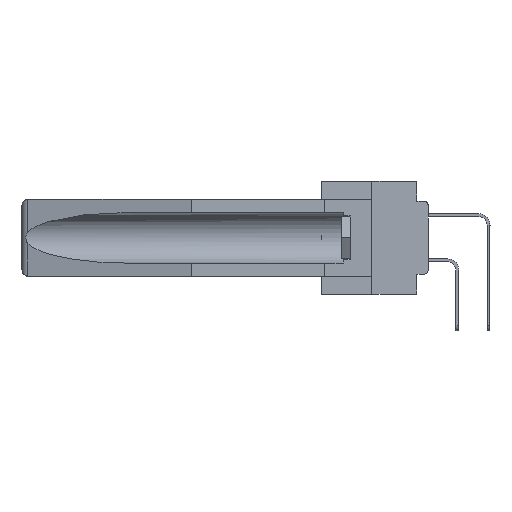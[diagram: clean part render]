
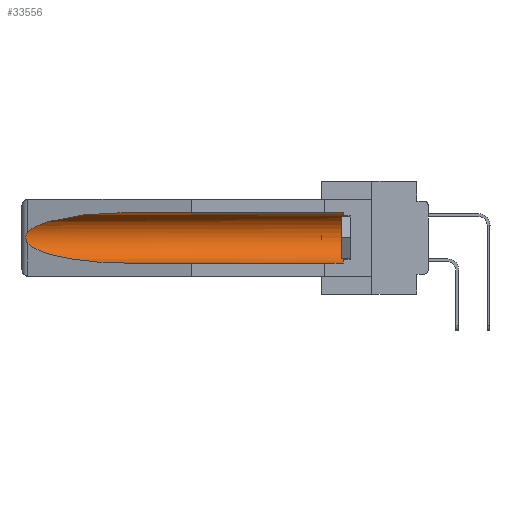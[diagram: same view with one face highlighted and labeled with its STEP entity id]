
A CAD part, left-side view. The second image highlights one B-rep face of the part: STEP entity #33556.
In plain terms, the highlighted cylindrical face has radius 2.857 mm (diameter 5.715 mm), a partial arc.
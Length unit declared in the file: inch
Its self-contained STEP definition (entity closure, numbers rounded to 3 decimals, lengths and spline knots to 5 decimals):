
#697 = DIRECTION ( 'NONE',  ( 0., 0., 1. ) ) ;
#1039 = CARTESIAN_POINT ( 'NONE',  ( 0.155, 1.07973, -0.284 ) ) ;
#2254 = CARTESIAN_POINT ( 'NONE',  ( 0.26537, 1.52718, -0.14972 ) ) ;
#2751 = VERTEX_POINT ( 'NONE', #34469 ) ;
#3448 = CARTESIAN_POINT ( 'NONE',  ( 0.2675, 1.53308, -0.16763 ) ) ;
#3685 = AXIS2_PLACEMENT_3D ( 'NONE', #16820, #39530, #697 ) ;
#3719 = CARTESIAN_POINT ( 'NONE',  ( 0.26654, 1.53092, -0.15636 ) ) ;
#5599 = CYLINDRICAL_SURFACE ( 'NONE', #23525, 0.1125 ) ;
#5653 = CARTESIAN_POINT ( 'NONE',  ( 0.155, -0.30754, -0.284 ) ) ;
#6281 = LINE ( 'NONE', #5653, #39744 ) ;
#6482 = CARTESIAN_POINT ( 'NONE',  ( 0.155, 1.07973, -0.284 ) ) ;
#7135 = VERTEX_POINT ( 'NONE', #21342 ) ;
#7260 = CARTESIAN_POINT ( 'NONE',  ( 0.26537, 1.52718, -0.19328 ) ) ;
#7741 = VERTEX_POINT ( 'NONE', #1039 ) ;
#11062 = EDGE_LOOP ( 'NONE', ( #20081, #21337, #25285, #20345, #12530, #34948 ) ) ;
#11138 =( BOUNDED_CURVE ( )  B_SPLINE_CURVE ( 3, ( #12547, #38806, #25921, #6482 ),
 .UNSPECIFIED., .F., .F. ) 
 B_SPLINE_CURVE_WITH_KNOTS ( ( 4, 4 ),
 ( 0.1948, 1.5708 ),
 .UNSPECIFIED. ) 
 CURVE ( )  GEOMETRIC_REPRESENTATION_ITEM ( )  RATIONAL_B_SPLINE_CURVE ( ( 1., 0.848, 0.848, 1. ) ) 
 REPRESENTATION_ITEM ( '' )  );
#11171 = CARTESIAN_POINT ( 'NONE',  ( 0.155, -0.30754, -0.059 ) ) ;
#11403 = EDGE_CURVE ( 'NONE', #7135, #7741, #11138, .T. ) ;
#12167 = CARTESIAN_POINT ( 'NONE',  ( 0.21114, 1.30732, -0.059 ) ) ;
#12530 = ORIENTED_EDGE ( 'NONE', *, *, #24722, .T. ) ;
#12547 = CARTESIAN_POINT ( 'NONE',  ( 0.26537, 1.52718, -0.19328 ) ) ;
#12862 = EDGE_CURVE ( 'NONE', #21431, #7741, #6281, .T. ) ;
#13477 = CARTESIAN_POINT ( 'NONE',  ( 0.2673, 1.53269, -0.17917 ) ) ;
#13538 = CIRCLE ( 'NONE', #3685, 0.1125 ) ;
#13752 = CARTESIAN_POINT ( 'NONE',  ( 0.26597, 1.52961, -0.15275 ) ) ;
#15125 = EDGE_CURVE ( 'NONE', #19023, #37343, #40006, .T. ) ;
#16593 = CARTESIAN_POINT ( 'NONE',  ( 0.2673, 1.5327, -0.16383 ) ) ;
#16713 = FACE_OUTER_BOUND ( 'NONE', #11062, .T. ) ;
#16739 = CARTESIAN_POINT ( 'NONE',  ( 0.2675, 1.53308, -0.17534 ) ) ;
#16820 = CARTESIAN_POINT ( 'NONE',  ( 0.155, 0.126, -0.1715 ) ) ;
#16988 = LINE ( 'NONE', #11171, #27691 ) ;
#18700 = DIRECTION ( 'NONE',  ( 0., 1., 0. ) ) ;
#18884 = CARTESIAN_POINT ( 'NONE',  ( 0.155, -0.30754, -0.1715 ) ) ;
#19023 = VERTEX_POINT ( 'NONE', #19279 ) ;
#19279 = CARTESIAN_POINT ( 'NONE',  ( 0.155, 1.07973, -0.059 ) ) ;
#20081 = ORIENTED_EDGE ( 'NONE', *, *, #15125, .T. ) ;
#20345 = ORIENTED_EDGE ( 'NONE', *, *, #12862, .F. ) ;
#21337 = ORIENTED_EDGE ( 'NONE', *, *, #33250, .T. ) ;
#21342 = CARTESIAN_POINT ( 'NONE',  ( 0.26537, 1.52718, -0.19328 ) ) ;
#21431 = VERTEX_POINT ( 'NONE', #39863 ) ;
#23031 = CARTESIAN_POINT ( 'NONE',  ( 0.26597, 1.5296, -0.19026 ) ) ;
#23298 = CARTESIAN_POINT ( 'NONE',  ( 0.26655, 1.53094, -0.18657 ) ) ;
#23525 = AXIS2_PLACEMENT_3D ( 'NONE', #18884, #34912, #41578 ) ;
#24722 = EDGE_CURVE ( 'NONE', #21431, #2751, #13538, .T. ) ;
#25285 = ORIENTED_EDGE ( 'NONE', *, *, #11403, .T. ) ;
#25401 = CARTESIAN_POINT ( 'NONE',  ( 0.155, 1.07973, -0.059 ) ) ;
#25921 = CARTESIAN_POINT ( 'NONE',  ( 0.21114, 1.30732, -0.284 ) ) ;
#27691 = VECTOR ( 'NONE', #33333, 39.37008 ) ;
#28647 = CARTESIAN_POINT ( 'NONE',  ( 0.26537, 1.52718, -0.14972 ) ) ;
#29894 = B_SPLINE_CURVE_WITH_KNOTS ( 'NONE', 3,
 ( #38616, #13752, #3719, #16593, #3448, #16739, #13477, #23298, #23031, #7260 ),
 .UNSPECIFIED., .F., .F.,
 ( 4, 2, 2, 2, 4 ),
 ( 0., 0.00029, 0.00058, 0.00087, 0.00117 ),
 .UNSPECIFIED. ) ;
#33250 = EDGE_CURVE ( 'NONE', #37343, #7135, #29894, .T. ) ;
#33333 = DIRECTION ( 'NONE',  ( 0., 1., 0. ) ) ;
#33556 = ADVANCED_FACE ( 'NONE', ( #16713 ), #5599, .F. ) ;
#34469 = CARTESIAN_POINT ( 'NONE',  ( 0.155, 0.126, -0.059 ) ) ;
#34912 = DIRECTION ( 'NONE',  ( 0., 1., 0. ) ) ;
#34948 = ORIENTED_EDGE ( 'NONE', *, *, #37000, .T. ) ;
#37000 = EDGE_CURVE ( 'NONE', #2751, #19023, #16988, .T. ) ;
#37343 = VERTEX_POINT ( 'NONE', #2254 ) ;
#38559 = CARTESIAN_POINT ( 'NONE',  ( 0.25451, 1.48313, -0.09465 ) ) ;
#38616 = CARTESIAN_POINT ( 'NONE',  ( 0.26537, 1.52718, -0.14972 ) ) ;
#38806 = CARTESIAN_POINT ( 'NONE',  ( 0.25451, 1.48313, -0.24835 ) ) ;
#39530 = DIRECTION ( 'NONE',  ( 0., -1., 0. ) ) ;
#39744 = VECTOR ( 'NONE', #18700, 39.37008 ) ;
#39863 = CARTESIAN_POINT ( 'NONE',  ( 0.155, 0.126, -0.284 ) ) ;
#40006 =( BOUNDED_CURVE ( )  B_SPLINE_CURVE ( 3, ( #25401, #12167, #38559, #28647 ),
 .UNSPECIFIED., .F., .F. ) 
 B_SPLINE_CURVE_WITH_KNOTS ( ( 4, 4 ),
 ( 4.71239, 6.08839 ),
 .UNSPECIFIED. ) 
 CURVE ( )  GEOMETRIC_REPRESENTATION_ITEM ( )  RATIONAL_B_SPLINE_CURVE ( ( 1., 0.848, 0.848, 1. ) ) 
 REPRESENTATION_ITEM ( '' )  );
#41578 = DIRECTION ( 'NONE',  ( 0., 0., 1. ) ) ;
